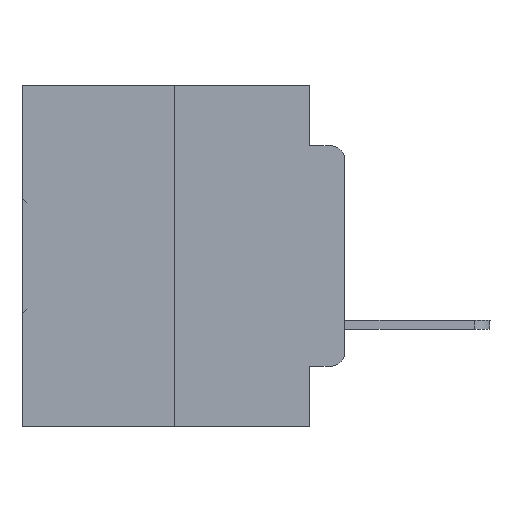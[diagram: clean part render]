
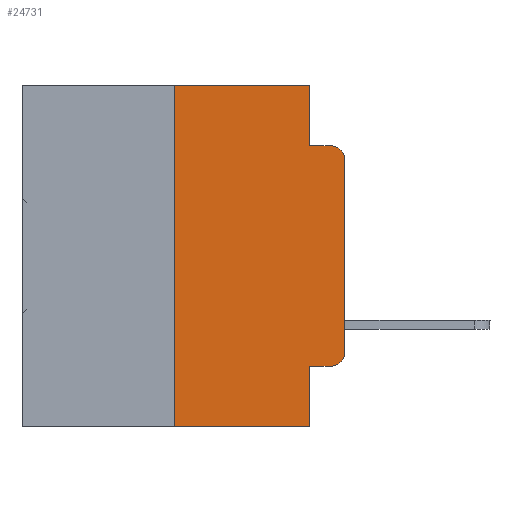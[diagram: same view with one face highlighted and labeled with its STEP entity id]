
A CAD part, left-side view. The second image highlights one B-rep face of the part: STEP entity #24731.
In plain terms, the highlighted planar face has unit normal (-1, 0, 0).
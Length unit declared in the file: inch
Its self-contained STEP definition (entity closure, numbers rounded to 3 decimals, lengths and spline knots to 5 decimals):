
#513 = VECTOR ( 'NONE', #23079, 39.37008 ) ;
#561 = CARTESIAN_POINT ( 'NONE',  ( 0., 0.25, 0. ) ) ;
#745 = LINE ( 'NONE', #829, #22234 ) ;
#829 = CARTESIAN_POINT ( 'NONE',  ( 0., 0.051, 0. ) ) ;
#1345 = VECTOR ( 'NONE', #30593, 39.37008 ) ;
#1630 = EDGE_CURVE ( 'NONE', #3680, #29553, #29084, .T. ) ;
#1793 = EDGE_CURVE ( 'NONE', #7732, #17958, #4871, .T. ) ;
#1938 = DIRECTION ( 'NONE',  ( 0., 0., 1. ) ) ;
#2624 = DIRECTION ( 'NONE',  ( -1., 0., 0. ) ) ;
#3661 = AXIS2_PLACEMENT_3D ( 'NONE', #14356, #17017, #22213 ) ;
#3680 = VERTEX_POINT ( 'NONE', #561 ) ;
#3935 = DIRECTION ( 'NONE',  ( 0., -1., 0. ) ) ;
#4125 = CARTESIAN_POINT ( 'NONE',  ( 0., 0.25, -0.5 ) ) ;
#4427 = VERTEX_POINT ( 'NONE', #31519 ) ;
#4431 = CIRCLE ( 'NONE', #23059, 0.02 ) ;
#4871 = LINE ( 'NONE', #24385, #16568 ) ;
#5685 = EDGE_CURVE ( 'NONE', #8484, #29373, #26867, .T. ) ;
#6385 = CARTESIAN_POINT ( 'NONE',  ( 0., 0.051, -0.0885 ) ) ;
#6608 = CARTESIAN_POINT ( 'NONE',  ( 0., 0., -0.3915 ) ) ;
#6707 = CARTESIAN_POINT ( 'NONE',  ( 0., 0., -0.1085 ) ) ;
#7704 = VERTEX_POINT ( 'NONE', #4125 ) ;
#7732 = VERTEX_POINT ( 'NONE', #6608 ) ;
#7958 = ORIENTED_EDGE ( 'NONE', *, *, #29760, .F. ) ;
#8063 = EDGE_CURVE ( 'NONE', #12419, #4427, #18401, .T. ) ;
#8484 = VERTEX_POINT ( 'NONE', #6385 ) ;
#8521 = ORIENTED_EDGE ( 'NONE', *, *, #31866, .F. ) ;
#8879 = DIRECTION ( 'NONE',  ( 0., -1., 0. ) ) ;
#9423 = DIRECTION ( 'NONE',  ( -1., 0., 0. ) ) ;
#9880 = CIRCLE ( 'NONE', #32437, 0.02 ) ;
#10184 = VECTOR ( 'NONE', #3935, 39.37008 ) ;
#10688 = EDGE_CURVE ( 'NONE', #7704, #4427, #20317, .T. ) ;
#11114 = CARTESIAN_POINT ( 'NONE',  ( 0., 0.473, 0. ) ) ;
#11313 = FACE_OUTER_BOUND ( 'NONE', #18188, .T. ) ;
#11781 = DIRECTION ( 'NONE',  ( 0., 0., -1. ) ) ;
#11942 = LINE ( 'NONE', #29764, #22500 ) ;
#12419 = VERTEX_POINT ( 'NONE', #18189 ) ;
#12818 = CARTESIAN_POINT ( 'NONE',  ( 0., 0.02, -0.0885 ) ) ;
#13345 = CARTESIAN_POINT ( 'NONE',  ( 0., 0.051, 0. ) ) ;
#13494 = DIRECTION ( 'NONE',  ( 0., 0., -1. ) ) ;
#14043 = EDGE_CURVE ( 'NONE', #12419, #22238, #11942, .T. ) ;
#14288 = ORIENTED_EDGE ( 'NONE', *, *, #8063, .F. ) ;
#14356 = CARTESIAN_POINT ( 'NONE',  ( 0., 0.473, 0. ) ) ;
#14596 = PLANE ( 'NONE',  #3661 ) ;
#16297 = LINE ( 'NONE', #25116, #1345 ) ;
#16568 = VECTOR ( 'NONE', #1938, 39.37008 ) ;
#17017 = DIRECTION ( 'NONE',  ( 1., 0., 0. ) ) ;
#17137 = CARTESIAN_POINT ( 'NONE',  ( 0., 0.051, 0. ) ) ;
#17958 = VERTEX_POINT ( 'NONE', #6707 ) ;
#18188 = EDGE_LOOP ( 'NONE', ( #18254, #18624, #18551, #8521, #19663, #7958, #22162, #14288, #28162, #29531 ) ) ;
#18189 = CARTESIAN_POINT ( 'NONE',  ( 0., 0.051, -0.4115 ) ) ;
#18216 = EDGE_CURVE ( 'NONE', #22238, #7732, #4431, .T. ) ;
#18254 = ORIENTED_EDGE ( 'NONE', *, *, #1793, .T. ) ;
#18401 = LINE ( 'NONE', #17137, #26512 ) ;
#18551 = ORIENTED_EDGE ( 'NONE', *, *, #5685, .F. ) ;
#18624 = ORIENTED_EDGE ( 'NONE', *, *, #22006, .T. ) ;
#19079 = CARTESIAN_POINT ( 'NONE',  ( 0., 0.473, -0.5 ) ) ;
#19663 = ORIENTED_EDGE ( 'NONE', *, *, #1630, .F. ) ;
#19813 = VECTOR ( 'NONE', #23812, 39.37008 ) ;
#20058 = DIRECTION ( 'NONE',  ( 0., 0., -1. ) ) ;
#20317 = LINE ( 'NONE', #19079, #10184 ) ;
#22006 = EDGE_CURVE ( 'NONE', #17958, #29373, #9880, .T. ) ;
#22162 = ORIENTED_EDGE ( 'NONE', *, *, #10688, .T. ) ;
#22213 = DIRECTION ( 'NONE',  ( 0., 0., -1. ) ) ;
#22234 = VECTOR ( 'NONE', #13494, 39.37008 ) ;
#22238 = VERTEX_POINT ( 'NONE', #25094 ) ;
#22500 = VECTOR ( 'NONE', #8879, 39.37008 ) ;
#23059 = AXIS2_PLACEMENT_3D ( 'NONE', #28175, #2624, #28289 ) ;
#23079 = DIRECTION ( 'NONE',  ( 0., -1., 0. ) ) ;
#23812 = DIRECTION ( 'NONE',  ( 0., -1., 0. ) ) ;
#24385 = CARTESIAN_POINT ( 'NONE',  ( 0., 0., 0. ) ) ;
#24731 = ADVANCED_FACE ( 'NONE', ( #11313 ), #14596, .F. ) ;
#25094 = CARTESIAN_POINT ( 'NONE',  ( 0., 0.02, -0.4115 ) ) ;
#25116 = CARTESIAN_POINT ( 'NONE',  ( 0., 0.25, 0. ) ) ;
#25986 = CARTESIAN_POINT ( 'NONE',  ( 0., 0.051, -0.0885 ) ) ;
#26512 = VECTOR ( 'NONE', #11781, 39.37008 ) ;
#26867 = LINE ( 'NONE', #25986, #513 ) ;
#28162 = ORIENTED_EDGE ( 'NONE', *, *, #14043, .T. ) ;
#28175 = CARTESIAN_POINT ( 'NONE',  ( 0., 0.02, -0.3915 ) ) ;
#28289 = DIRECTION ( 'NONE',  ( 0., 0., -1. ) ) ;
#29084 = LINE ( 'NONE', #11114, #19813 ) ;
#29373 = VERTEX_POINT ( 'NONE', #12818 ) ;
#29531 = ORIENTED_EDGE ( 'NONE', *, *, #18216, .T. ) ;
#29553 = VERTEX_POINT ( 'NONE', #13345 ) ;
#29760 = EDGE_CURVE ( 'NONE', #7704, #3680, #16297, .T. ) ;
#29764 = CARTESIAN_POINT ( 'NONE',  ( 0., 0.051, -0.4115 ) ) ;
#30315 = CARTESIAN_POINT ( 'NONE',  ( 0., 0.02, -0.1085 ) ) ;
#30593 = DIRECTION ( 'NONE',  ( 0., 0., 1. ) ) ;
#31519 = CARTESIAN_POINT ( 'NONE',  ( 0., 0.051, -0.5 ) ) ;
#31866 = EDGE_CURVE ( 'NONE', #29553, #8484, #745, .T. ) ;
#32437 = AXIS2_PLACEMENT_3D ( 'NONE', #30315, #9423, #20058 ) ;
